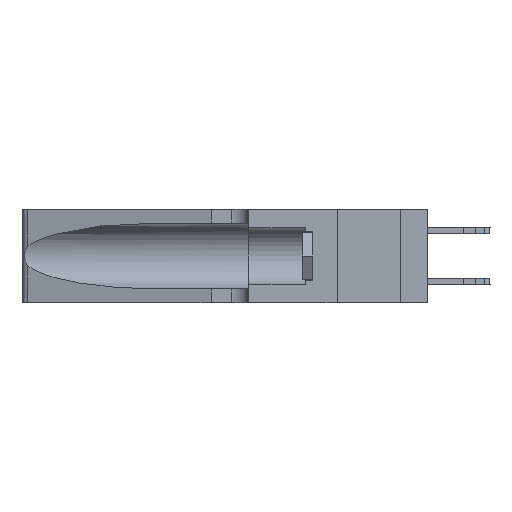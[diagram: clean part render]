
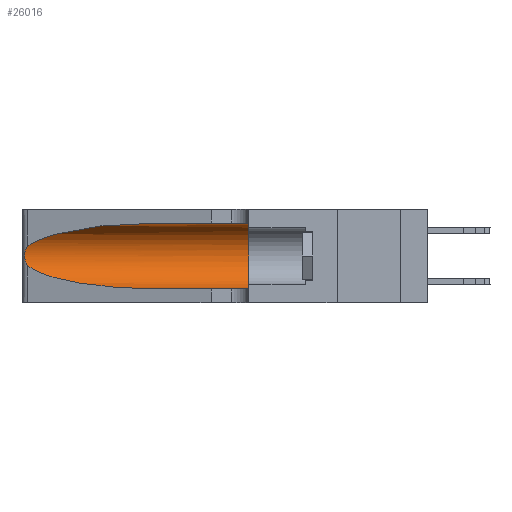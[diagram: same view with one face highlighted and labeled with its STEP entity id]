
A CAD part, left-side view. The second image highlights one B-rep face of the part: STEP entity #26016.
In plain terms, the highlighted cylindrical face has radius 3.308 mm (diameter 6.617 mm), a partial arc.
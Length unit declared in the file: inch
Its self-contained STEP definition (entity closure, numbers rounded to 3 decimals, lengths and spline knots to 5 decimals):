
#375 = EDGE_CURVE ( 'NONE', #10581, #24338, #4508, .T. ) ;
#1644 = EDGE_CURVE ( 'NONE', #24338, #26260, #15772, .T. ) ;
#2231 = CARTESIAN_POINT ( 'NONE',  ( 0.25856, 1.23593, 0.16098 ) ) ;
#2328 = CARTESIAN_POINT ( 'NONE',  ( 0.26075, 1.23896, 0.19203 ) ) ;
#2917 = CARTESIAN_POINT ( 'NONE',  ( 0.2373, 1.15595, 0.08982 ) ) ;
#3277 = CARTESIAN_POINT ( 'NONE',  ( 0.25487, 1.22718, 0.14631 ) ) ;
#3980 = DIRECTION ( 'NONE',  ( 0., 1., 0. ) ) ;
#4011 = VECTOR ( 'NONE', #4047, 39.37008 ) ;
#4047 = DIRECTION ( 'NONE',  ( 0., -1., 0. ) ) ;
#4048 = EDGE_CURVE ( 'NONE', #10581, #8083, #23085, .T. ) ;
#4508 =( BOUNDED_CURVE ( )  B_SPLINE_CURVE ( 3, ( #25889, #8375, #28311, #13869 ),
 .UNSPECIFIED., .F., .T. ) 
 B_SPLINE_CURVE_WITH_KNOTS ( ( 4, 4 ),
 ( 1.5708, 2.84003 ),
 .UNSPECIFIED. ) 
 CURVE ( )  GEOMETRIC_REPRESENTATION_ITEM ( )  RATIONAL_B_SPLINE_CURVE ( ( 1., 0.87, 0.87, 1. ) ) 
 REPRESENTATION_ITEM ( '' )  );
#4546 = CARTESIAN_POINT ( 'NONE',  ( 0.25787, 1.23484, 0.2124 ) ) ;
#4980 = AXIS2_PLACEMENT_3D ( 'NONE', #10680, #3980, #13524 ) ;
#5059 = CARTESIAN_POINT ( 'NONE',  ( 0.1305, 0.72297, 0.05475 ) ) ;
#5160 = CARTESIAN_POINT ( 'NONE',  ( 0.1305, 0.35, 0.31525 ) ) ;
#5164 = CARTESIAN_POINT ( 'NONE',  ( 0.25487, 1.22718, 0.14631 ) ) ;
#6246 = EDGE_CURVE ( 'NONE', #15119, #29743, #10116, .T. ) ;
#6730 = ORIENTED_EDGE ( 'NONE', *, *, #375, .T. ) ;
#8083 = VERTEX_POINT ( 'NONE', #5160 ) ;
#8375 = CARTESIAN_POINT ( 'NONE',  ( 0.18966, 0.96281, 0.31525 ) ) ;
#9293 = AXIS2_PLACEMENT_3D ( 'NONE', #16783, #11848, #17075 ) ;
#9776 = CARTESIAN_POINT ( 'NONE',  ( 0.25639, 1.23184, 0.21858 ) ) ;
#9876 = FACE_OUTER_BOUND ( 'NONE', #20968, .T. ) ;
#10116 = LINE ( 'NONE', #30971, #4011 ) ;
#10581 = VERTEX_POINT ( 'NONE', #15794 ) ;
#10680 = CARTESIAN_POINT ( 'NONE',  ( 0.1305, 0.35, 0.185 ) ) ;
#11209 = EDGE_CURVE ( 'NONE', #8083, #29743, #20956, .T. ) ;
#11848 = DIRECTION ( 'NONE',  ( 0., -1., 0. ) ) ;
#12091 = CARTESIAN_POINT ( 'NONE',  ( 0.26018, 1.23835, 0.19895 ) ) ;
#12335 = ORIENTED_EDGE ( 'NONE', *, *, #11209, .F. ) ;
#12780 = CARTESIAN_POINT ( 'NONE',  ( 0.18966, 0.96281, 0.05475 ) ) ;
#13524 = DIRECTION ( 'NONE',  ( 0., 0., 1. ) ) ;
#13869 = CARTESIAN_POINT ( 'NONE',  ( 0.25487, 1.22718, 0.22369 ) ) ;
#14310 = CARTESIAN_POINT ( 'NONE',  ( 0.25487, 1.22718, 0.22369 ) ) ;
#14519 = CARTESIAN_POINT ( 'NONE',  ( 0.25555, 1.22993, 0.14849 ) ) ;
#15119 = VERTEX_POINT ( 'NONE', #15352 ) ;
#15352 = CARTESIAN_POINT ( 'NONE',  ( 0.1305, 0.72297, 0.05475 ) ) ;
#15772 = B_SPLINE_CURVE_WITH_KNOTS ( 'NONE', 3,
 ( #14310, #19022, #9776, #4546, #28877, #12091, #2328, #31270, #16816, #2231, #19217, #28973, #14519, #16717 ),
 .UNSPECIFIED., .F., .F.,
 ( 4, 2, 2, 2, 2, 2, 4 ),
 ( 0., 0.00027, 0.00053, 0.00107, 0.0016, 0.00187, 0.00214 ),
 .UNSPECIFIED. ) ;
#15794 = CARTESIAN_POINT ( 'NONE',  ( 0.1305, 0.72297, 0.31525 ) ) ;
#16637 = ORIENTED_EDGE ( 'NONE', *, *, #4048, .F. ) ;
#16678 = VECTOR ( 'NONE', #16679, 39.37008 ) ;
#16679 = DIRECTION ( 'NONE',  ( 0., -1., 0. ) ) ;
#16717 = CARTESIAN_POINT ( 'NONE',  ( 0.25487, 1.22718, 0.14631 ) ) ;
#16783 = CARTESIAN_POINT ( 'NONE',  ( 0.1305, 1.61858, 0.185 ) ) ;
#16816 = CARTESIAN_POINT ( 'NONE',  ( 0.26017, 1.23833, 0.17102 ) ) ;
#17075 = DIRECTION ( 'NONE',  ( 0., 0., -1. ) ) ;
#19022 = CARTESIAN_POINT ( 'NONE',  ( 0.25555, 1.22994, 0.2215 ) ) ;
#19217 = CARTESIAN_POINT ( 'NONE',  ( 0.25789, 1.23486, 0.15765 ) ) ;
#20915 = ORIENTED_EDGE ( 'NONE', *, *, #29109, .T. ) ;
#20956 = CIRCLE ( 'NONE', #4980, 0.13025 ) ;
#20968 = EDGE_LOOP ( 'NONE', ( #6730, #26028, #20915, #26439, #12335, #16637 ) ) ;
#23085 = LINE ( 'NONE', #28945, #16678 ) ;
#24338 = VERTEX_POINT ( 'NONE', #27172 ) ;
#25889 = CARTESIAN_POINT ( 'NONE',  ( 0.1305, 0.72297, 0.31525 ) ) ;
#26016 = ADVANCED_FACE ( 'NONE', ( #9876 ), #29834, .F. ) ;
#26028 = ORIENTED_EDGE ( 'NONE', *, *, #1644, .T. ) ;
#26260 = VERTEX_POINT ( 'NONE', #3277 ) ;
#26439 = ORIENTED_EDGE ( 'NONE', *, *, #6246, .T. ) ;
#26517 = CARTESIAN_POINT ( 'NONE',  ( 0.1305, 0.35, 0.05475 ) ) ;
#27172 = CARTESIAN_POINT ( 'NONE',  ( 0.25487, 1.22718, 0.22369 ) ) ;
#28311 = CARTESIAN_POINT ( 'NONE',  ( 0.2373, 1.15595, 0.28018 ) ) ;
#28877 = CARTESIAN_POINT ( 'NONE',  ( 0.25854, 1.2359, 0.20912 ) ) ;
#28945 = CARTESIAN_POINT ( 'NONE',  ( 0.1305, 1.61858, 0.31525 ) ) ;
#28973 = CARTESIAN_POINT ( 'NONE',  ( 0.25639, 1.23186, 0.15144 ) ) ;
#29109 = EDGE_CURVE ( 'NONE', #26260, #15119, #29470, .T. ) ;
#29470 =( BOUNDED_CURVE ( )  B_SPLINE_CURVE ( 3, ( #5164, #2917, #12780, #5059 ),
 .UNSPECIFIED., .F., .F. ) 
 B_SPLINE_CURVE_WITH_KNOTS ( ( 4, 4 ),
 ( 3.44316, 4.71239 ),
 .UNSPECIFIED. ) 
 CURVE ( )  GEOMETRIC_REPRESENTATION_ITEM ( )  RATIONAL_B_SPLINE_CURVE ( ( 1., 0.87, 0.87, 1. ) ) 
 REPRESENTATION_ITEM ( '' )  );
#29743 = VERTEX_POINT ( 'NONE', #26517 ) ;
#29834 = CYLINDRICAL_SURFACE ( 'NONE', #9293, 0.13025 ) ;
#30971 = CARTESIAN_POINT ( 'NONE',  ( 0.1305, 1.61858, 0.05475 ) ) ;
#31270 = CARTESIAN_POINT ( 'NONE',  ( 0.26075, 1.23896, 0.178 ) ) ;
